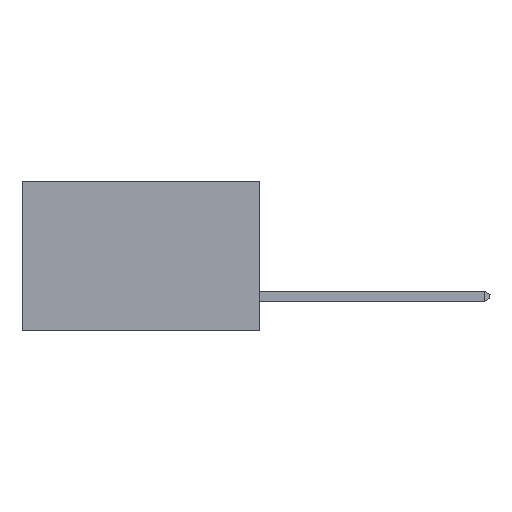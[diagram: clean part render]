
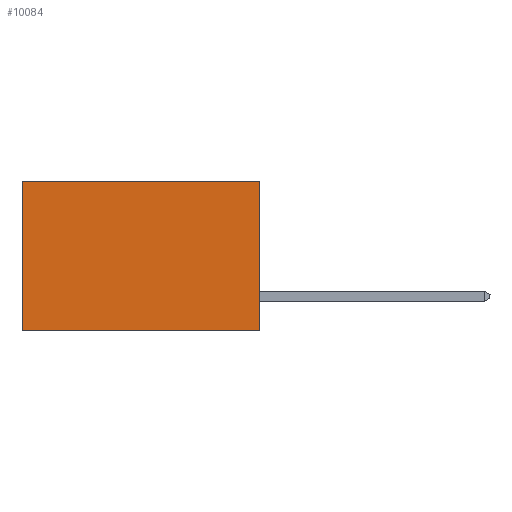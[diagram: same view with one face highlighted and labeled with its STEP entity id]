
A CAD part, left-side view. The second image highlights one B-rep face of the part: STEP entity #10084.
In plain terms, the highlighted planar face has unit normal (-1, 0, 0).
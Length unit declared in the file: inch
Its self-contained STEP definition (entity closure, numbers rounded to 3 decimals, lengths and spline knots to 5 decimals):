
#213 = CARTESIAN_POINT ( 'NONE',  ( 0.277, 0.59, -0.37 ) ) ;
#1678 = VERTEX_POINT ( 'NONE', #10820 ) ;
#1911 = EDGE_CURVE ( 'NONE', #1678, #4607, #2404, .T. ) ;
#2290 = CARTESIAN_POINT ( 'NONE',  ( 0.277, 0., -0.37 ) ) ;
#2404 = LINE ( 'NONE', #8767, #4704 ) ;
#2899 = VECTOR ( 'NONE', #11314, 39.37008 ) ;
#3137 = VERTEX_POINT ( 'NONE', #213 ) ;
#3772 = VECTOR ( 'NONE', #6824, 39.37008 ) ;
#3784 = CARTESIAN_POINT ( 'NONE',  ( 0.277, 0., -0.37 ) ) ;
#4470 = EDGE_CURVE ( 'NONE', #1678, #5349, #5462, .T. ) ;
#4607 = VERTEX_POINT ( 'NONE', #8559 ) ;
#4704 = VECTOR ( 'NONE', #6990, 39.37008 ) ;
#5042 = FACE_OUTER_BOUND ( 'NONE', #9758, .T. ) ;
#5227 = ORIENTED_EDGE ( 'NONE', *, *, #7946, .T. ) ;
#5248 = DIRECTION ( 'NONE',  ( 1., 0., 0. ) ) ;
#5349 = VERTEX_POINT ( 'NONE', #9278 ) ;
#5462 = LINE ( 'NONE', #3784, #2899 ) ;
#5688 = VECTOR ( 'NONE', #9598, 39.37008 ) ;
#5901 = ORIENTED_EDGE ( 'NONE', *, *, #6397, .F. ) ;
#6032 = LINE ( 'NONE', #6826, #3772 ) ;
#6286 = ORIENTED_EDGE ( 'NONE', *, *, #4470, .F. ) ;
#6397 = EDGE_CURVE ( 'NONE', #5349, #3137, #6032, .T. ) ;
#6824 = DIRECTION ( 'NONE',  ( 0., 1., 0. ) ) ;
#6826 = CARTESIAN_POINT ( 'NONE',  ( 0.277, 0., -0.37 ) ) ;
#6990 = DIRECTION ( 'NONE',  ( 0., 1., 0. ) ) ;
#7946 = EDGE_CURVE ( 'NONE', #4607, #3137, #10973, .T. ) ;
#8559 = CARTESIAN_POINT ( 'NONE',  ( 0.277, 0.59, 0. ) ) ;
#8767 = CARTESIAN_POINT ( 'NONE',  ( 0.277, 0., 0. ) ) ;
#9278 = CARTESIAN_POINT ( 'NONE',  ( 0.277, 0., -0.37 ) ) ;
#9598 = DIRECTION ( 'NONE',  ( 0., 0., -1. ) ) ;
#9670 = CARTESIAN_POINT ( 'NONE',  ( 0.277, 0.59, -0.37 ) ) ;
#9758 = EDGE_LOOP ( 'NONE', ( #5227, #5901, #6286, #11450 ) ) ;
#10084 = ADVANCED_FACE ( 'NONE', ( #5042 ), #10624, .F. ) ;
#10624 = PLANE ( 'NONE',  #11962 ) ;
#10820 = CARTESIAN_POINT ( 'NONE',  ( 0.277, 0., 0. ) ) ;
#10973 = LINE ( 'NONE', #9670, #5688 ) ;
#11314 = DIRECTION ( 'NONE',  ( 0., 0., -1. ) ) ;
#11450 = ORIENTED_EDGE ( 'NONE', *, *, #1911, .T. ) ;
#11508 = DIRECTION ( 'NONE',  ( 0., 0., -1. ) ) ;
#11962 = AXIS2_PLACEMENT_3D ( 'NONE', #2290, #5248, #11508 ) ;
